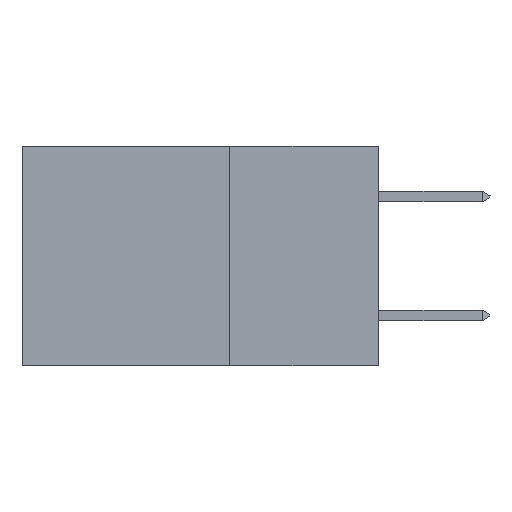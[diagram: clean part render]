
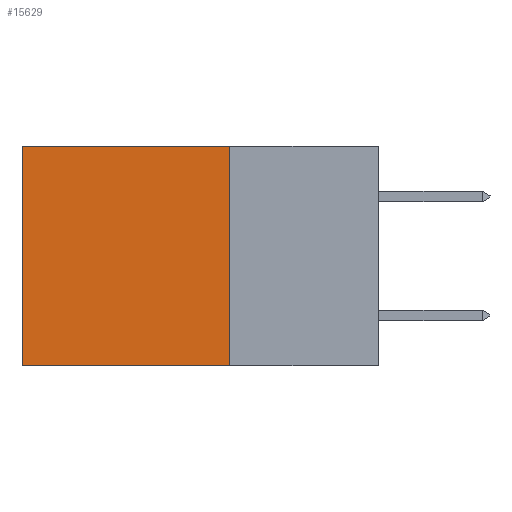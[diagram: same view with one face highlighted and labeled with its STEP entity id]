
A CAD part, left-side view. The second image highlights one B-rep face of the part: STEP entity #15629.
In plain terms, the highlighted planar face has unit normal (-1, 0, 0).
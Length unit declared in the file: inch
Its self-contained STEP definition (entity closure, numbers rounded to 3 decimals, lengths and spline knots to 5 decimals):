
#244 = CARTESIAN_POINT ( 'NONE',  ( 0.2615, 0.6, -0.37 ) ) ;
#308 = DIRECTION ( 'NONE',  ( 0., 0., -1. ) ) ;
#609 = EDGE_CURVE ( 'NONE', #8398, #1765, #18674, .T. ) ;
#749 = VECTOR ( 'NONE', #23269, 39.37008 ) ;
#968 = LINE ( 'NONE', #23328, #17265 ) ;
#1765 = VERTEX_POINT ( 'NONE', #3109 ) ;
#1807 = VECTOR ( 'NONE', #6197, 39.37008 ) ;
#2033 = ORIENTED_EDGE ( 'NONE', *, *, #609, .F. ) ;
#2048 = CARTESIAN_POINT ( 'NONE',  ( 0.2615, 0.25, -0.37 ) ) ;
#3109 = CARTESIAN_POINT ( 'NONE',  ( 0.2615, 0.25, -0.37 ) ) ;
#3579 = LINE ( 'NONE', #15155, #749 ) ;
#4603 = ORIENTED_EDGE ( 'NONE', *, *, #24875, .T. ) ;
#5115 = DIRECTION ( 'NONE',  ( 0., 1., 0. ) ) ;
#5549 = EDGE_CURVE ( 'NONE', #1765, #9207, #26151, .T. ) ;
#6197 = DIRECTION ( 'NONE',  ( 0., 1., 0. ) ) ;
#8398 = VERTEX_POINT ( 'NONE', #19600 ) ;
#8469 = FACE_OUTER_BOUND ( 'NONE', #11849, .T. ) ;
#9207 = VERTEX_POINT ( 'NONE', #244 ) ;
#10369 = ORIENTED_EDGE ( 'NONE', *, *, #5549, .F. ) ;
#10582 = CARTESIAN_POINT ( 'NONE',  ( 0.2615, 0.25, -0.37 ) ) ;
#11796 = VECTOR ( 'NONE', #308, 39.37008 ) ;
#11849 = EDGE_LOOP ( 'NONE', ( #21174, #10369, #2033, #4603 ) ) ;
#11933 = EDGE_CURVE ( 'NONE', #25446, #9207, #3579, .T. ) ;
#12436 = DIRECTION ( 'NONE',  ( 0., 0., -1. ) ) ;
#12696 = PLANE ( 'NONE',  #24254 ) ;
#15155 = CARTESIAN_POINT ( 'NONE',  ( 0.2615, 0.6, -0.37 ) ) ;
#15629 = ADVANCED_FACE ( 'NONE', ( #8469 ), #12696, .F. ) ;
#15958 = CARTESIAN_POINT ( 'NONE',  ( 0.2615, 0.6, 0. ) ) ;
#17265 = VECTOR ( 'NONE', #5115, 39.37008 ) ;
#18674 = LINE ( 'NONE', #2048, #11796 ) ;
#18805 = DIRECTION ( 'NONE',  ( 1., 0., 0. ) ) ;
#19600 = CARTESIAN_POINT ( 'NONE',  ( 0.2615, 0.25, 0. ) ) ;
#21174 = ORIENTED_EDGE ( 'NONE', *, *, #11933, .T. ) ;
#22273 = CARTESIAN_POINT ( 'NONE',  ( 0.2615, 0.25, -0.37 ) ) ;
#23269 = DIRECTION ( 'NONE',  ( 0., 0., -1. ) ) ;
#23328 = CARTESIAN_POINT ( 'NONE',  ( 0.2615, 0.25, 0. ) ) ;
#24254 = AXIS2_PLACEMENT_3D ( 'NONE', #10582, #18805, #12436 ) ;
#24875 = EDGE_CURVE ( 'NONE', #8398, #25446, #968, .T. ) ;
#25446 = VERTEX_POINT ( 'NONE', #15958 ) ;
#26151 = LINE ( 'NONE', #22273, #1807 ) ;
